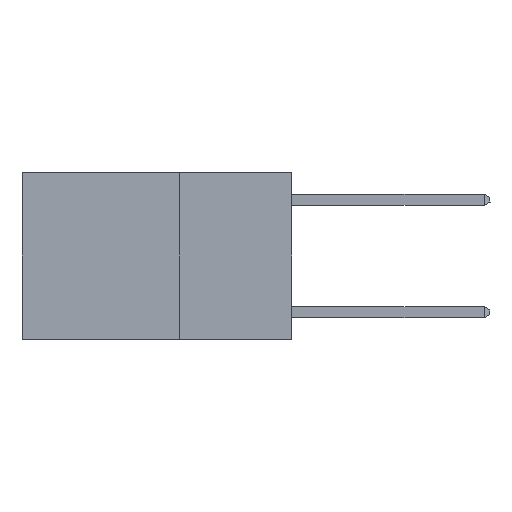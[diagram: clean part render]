
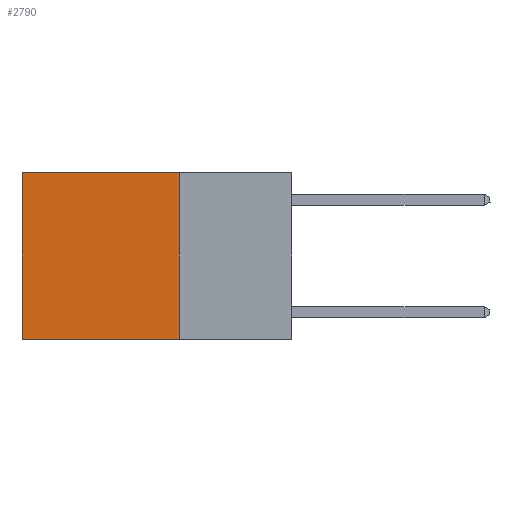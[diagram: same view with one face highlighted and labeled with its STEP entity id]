
A CAD part, left-side view. The second image highlights one B-rep face of the part: STEP entity #2790.
In plain terms, the highlighted planar face has unit normal (-1, 0, 0).
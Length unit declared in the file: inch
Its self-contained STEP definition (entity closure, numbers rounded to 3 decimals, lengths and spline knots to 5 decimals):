
#735 = CARTESIAN_POINT ( 'NONE',  ( 0.2625, 0.25, 0. ) ) ;
#1016 = LINE ( 'NONE', #8961, #13235 ) ;
#1541 = FACE_OUTER_BOUND ( 'NONE', #9053, .T. ) ;
#2790 = ADVANCED_FACE ( 'NONE', ( #1541 ), #10251, .F. ) ;
#3722 = VERTEX_POINT ( 'NONE', #9594 ) ;
#4051 = VECTOR ( 'NONE', #6277, 39.37008 ) ;
#4478 = VECTOR ( 'NONE', #12726, 39.37008 ) ;
#4481 = LINE ( 'NONE', #14169, #4051 ) ;
#4888 = VERTEX_POINT ( 'NONE', #8467 ) ;
#5434 = CARTESIAN_POINT ( 'NONE',  ( 0.2625, 0.25, 0. ) ) ;
#5451 = CARTESIAN_POINT ( 'NONE',  ( 0.2625, 0.25, 0. ) ) ;
#5695 = DIRECTION ( 'NONE',  ( 1., 0., 0. ) ) ;
#5945 = EDGE_CURVE ( 'NONE', #4888, #11872, #4481, .T. ) ;
#6277 = DIRECTION ( 'NONE',  ( 0., 1., 0. ) ) ;
#6544 = DIRECTION ( 'NONE',  ( 0., 1., 0. ) ) ;
#6631 = ORIENTED_EDGE ( 'NONE', *, *, #8823, .T. ) ;
#6759 = CARTESIAN_POINT ( 'NONE',  ( 0.2625, 0.6, -0.37 ) ) ;
#6864 = ORIENTED_EDGE ( 'NONE', *, *, #5945, .F. ) ;
#7121 = ORIENTED_EDGE ( 'NONE', *, *, #12474, .F. ) ;
#7307 = ORIENTED_EDGE ( 'NONE', *, *, #7683, .T. ) ;
#7683 = EDGE_CURVE ( 'NONE', #10303, #3722, #12040, .T. ) ;
#8467 = CARTESIAN_POINT ( 'NONE',  ( 0.2625, 0.25, -0.37 ) ) ;
#8823 = EDGE_CURVE ( 'NONE', #3722, #11872, #1016, .T. ) ;
#8860 = VECTOR ( 'NONE', #6544, 39.37008 ) ;
#8961 = CARTESIAN_POINT ( 'NONE',  ( 0.2625, 0.6, 0. ) ) ;
#9053 = EDGE_LOOP ( 'NONE', ( #6631, #6864, #7121, #7307 ) ) ;
#9089 = DIRECTION ( 'NONE',  ( 0., 0., -1. ) ) ;
#9186 = AXIS2_PLACEMENT_3D ( 'NONE', #735, #5695, #9089 ) ;
#9594 = CARTESIAN_POINT ( 'NONE',  ( 0.2625, 0.6, 0. ) ) ;
#10251 = PLANE ( 'NONE',  #9186 ) ;
#10303 = VERTEX_POINT ( 'NONE', #5434 ) ;
#10984 = LINE ( 'NONE', #11571, #4478 ) ;
#11571 = CARTESIAN_POINT ( 'NONE',  ( 0.2625, 0.25, 0. ) ) ;
#11872 = VERTEX_POINT ( 'NONE', #6759 ) ;
#12040 = LINE ( 'NONE', #5451, #8860 ) ;
#12474 = EDGE_CURVE ( 'NONE', #10303, #4888, #10984, .T. ) ;
#12726 = DIRECTION ( 'NONE',  ( 0., 0., -1. ) ) ;
#13235 = VECTOR ( 'NONE', #13634, 39.37008 ) ;
#13634 = DIRECTION ( 'NONE',  ( 0., 0., -1. ) ) ;
#14169 = CARTESIAN_POINT ( 'NONE',  ( 0.2625, 0.25, -0.37 ) ) ;
